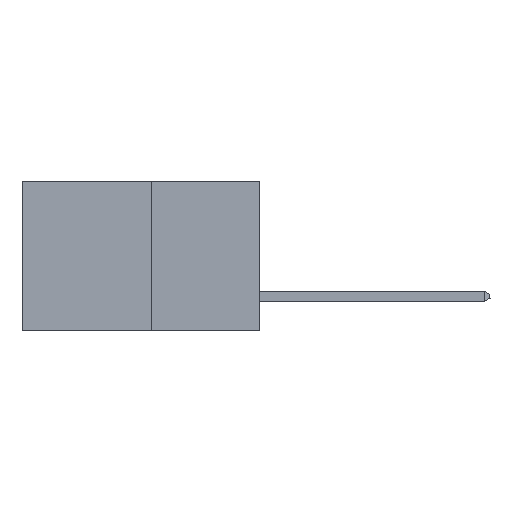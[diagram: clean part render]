
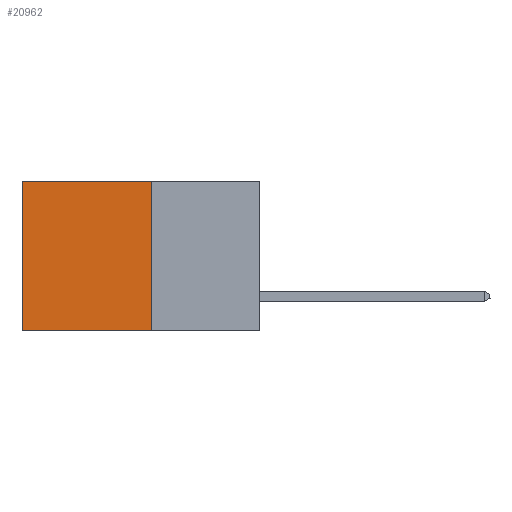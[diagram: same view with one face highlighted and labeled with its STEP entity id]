
A CAD part, left-side view. The second image highlights one B-rep face of the part: STEP entity #20962.
In plain terms, the highlighted planar face has unit normal (-1, 0, 0).
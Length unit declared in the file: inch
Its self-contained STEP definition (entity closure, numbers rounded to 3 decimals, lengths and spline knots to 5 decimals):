
#385 = LINE ( 'NONE', #24056, #24935 ) ;
#2018 = DIRECTION ( 'NONE',  ( 0., 0., -1. ) ) ;
#2672 = EDGE_CURVE ( 'NONE', #24184, #3569, #385, .T. ) ;
#2764 = CARTESIAN_POINT ( 'NONE',  ( 0.277, 0.27, -0.37 ) ) ;
#2935 = VECTOR ( 'NONE', #4407, 39.37008 ) ;
#3569 = VERTEX_POINT ( 'NONE', #21849 ) ;
#4407 = DIRECTION ( 'NONE',  ( 0., 0., -1. ) ) ;
#4496 = ORIENTED_EDGE ( 'NONE', *, *, #2672, .F. ) ;
#4904 = DIRECTION ( 'NONE',  ( 0., 0., -1. ) ) ;
#4985 = FACE_OUTER_BOUND ( 'NONE', #17522, .T. ) ;
#5307 = LINE ( 'NONE', #19200, #17271 ) ;
#5385 = EDGE_CURVE ( 'NONE', #12276, #27800, #28949, .T. ) ;
#8760 = EDGE_CURVE ( 'NONE', #12276, #24184, #15670, .T. ) ;
#8957 = ORIENTED_EDGE ( 'NONE', *, *, #5385, .T. ) ;
#9330 = CARTESIAN_POINT ( 'NONE',  ( 0.277, 0.27, 0. ) ) ;
#10304 = VECTOR ( 'NONE', #16391, 39.37008 ) ;
#11640 = PLANE ( 'NONE',  #13128 ) ;
#12276 = VERTEX_POINT ( 'NONE', #9330 ) ;
#13128 = AXIS2_PLACEMENT_3D ( 'NONE', #27967, #16352, #2018 ) ;
#15670 = LINE ( 'NONE', #23323, #2935 ) ;
#15796 = ORIENTED_EDGE ( 'NONE', *, *, #25347, .T. ) ;
#16290 = CARTESIAN_POINT ( 'NONE',  ( 0.277, 0.27, 0. ) ) ;
#16352 = DIRECTION ( 'NONE',  ( 1., 0., 0. ) ) ;
#16391 = DIRECTION ( 'NONE',  ( 0., 1., 0. ) ) ;
#17271 = VECTOR ( 'NONE', #4904, 39.37008 ) ;
#17522 = EDGE_LOOP ( 'NONE', ( #15796, #4496, #23433, #8957 ) ) ;
#19200 = CARTESIAN_POINT ( 'NONE',  ( 0.277, 0.59, -0.37 ) ) ;
#20962 = ADVANCED_FACE ( 'NONE', ( #4985 ), #11640, .F. ) ;
#21849 = CARTESIAN_POINT ( 'NONE',  ( 0.277, 0.59, -0.37 ) ) ;
#23323 = CARTESIAN_POINT ( 'NONE',  ( 0.277, 0.27, -0.37 ) ) ;
#23433 = ORIENTED_EDGE ( 'NONE', *, *, #8760, .F. ) ;
#24056 = CARTESIAN_POINT ( 'NONE',  ( 0.277, 0.27, -0.37 ) ) ;
#24184 = VERTEX_POINT ( 'NONE', #2764 ) ;
#24185 = DIRECTION ( 'NONE',  ( 0., 1., 0. ) ) ;
#24935 = VECTOR ( 'NONE', #24185, 39.37008 ) ;
#25347 = EDGE_CURVE ( 'NONE', #27800, #3569, #5307, .T. ) ;
#27783 = CARTESIAN_POINT ( 'NONE',  ( 0.277, 0.59, 0. ) ) ;
#27800 = VERTEX_POINT ( 'NONE', #27783 ) ;
#27967 = CARTESIAN_POINT ( 'NONE',  ( 0.277, 0.27, -0.37 ) ) ;
#28949 = LINE ( 'NONE', #16290, #10304 ) ;
